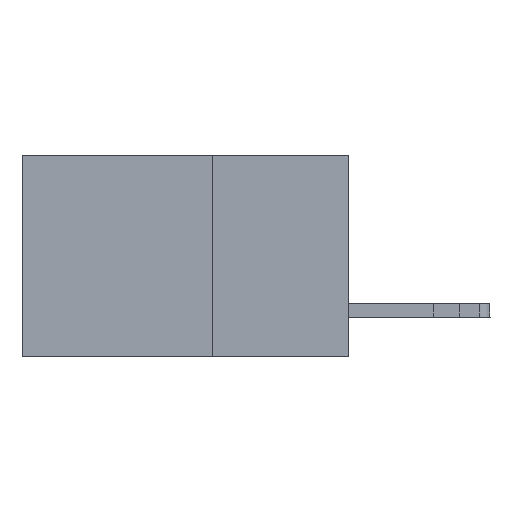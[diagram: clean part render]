
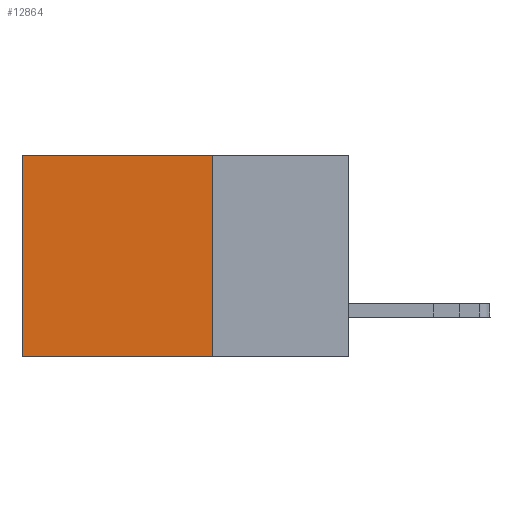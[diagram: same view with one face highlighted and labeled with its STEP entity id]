
A CAD part, left-side view. The second image highlights one B-rep face of the part: STEP entity #12864.
In plain terms, the highlighted planar face has unit normal (-1, 0, 0).
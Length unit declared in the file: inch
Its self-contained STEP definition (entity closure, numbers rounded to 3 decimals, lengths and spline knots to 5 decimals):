
#152 = CARTESIAN_POINT ( 'NONE',  ( 0.298, 0.25, 0. ) ) ;
#341 = DIRECTION ( 'NONE',  ( 0., 1., 0. ) ) ;
#676 = EDGE_CURVE ( 'NONE', #10019, #4765, #17692, .T. ) ;
#2193 = VECTOR ( 'NONE', #7711, 39.37008 ) ;
#2790 = EDGE_CURVE ( 'NONE', #4765, #21662, #24842, .T. ) ;
#4489 = EDGE_LOOP ( 'NONE', ( #12050, #15477, #16972, #23974 ) ) ;
#4526 = AXIS2_PLACEMENT_3D ( 'NONE', #23938, #21741, #7765 ) ;
#4765 = VERTEX_POINT ( 'NONE', #11971 ) ;
#5808 = EDGE_CURVE ( 'NONE', #10019, #13779, #13981, .T. ) ;
#6183 = CARTESIAN_POINT ( 'NONE',  ( 0.298, 0.6, -0.37 ) ) ;
#6931 = LINE ( 'NONE', #18487, #7171 ) ;
#7171 = VECTOR ( 'NONE', #16794, 39.37008 ) ;
#7711 = DIRECTION ( 'NONE',  ( 0., 0., -1. ) ) ;
#7765 = DIRECTION ( 'NONE',  ( 0., 0., -1. ) ) ;
#10019 = VERTEX_POINT ( 'NONE', #21011 ) ;
#11971 = CARTESIAN_POINT ( 'NONE',  ( 0.298, 0.25, -0.37 ) ) ;
#12050 = ORIENTED_EDGE ( 'NONE', *, *, #24105, .T. ) ;
#12864 = ADVANCED_FACE ( 'NONE', ( #16037 ), #25641, .F. ) ;
#13779 = VERTEX_POINT ( 'NONE', #22524 ) ;
#13981 = LINE ( 'NONE', #20196, #16504 ) ;
#15477 = ORIENTED_EDGE ( 'NONE', *, *, #2790, .F. ) ;
#16037 = FACE_OUTER_BOUND ( 'NONE', #4489, .T. ) ;
#16409 = VECTOR ( 'NONE', #17212, 39.37008 ) ;
#16504 = VECTOR ( 'NONE', #341, 39.37008 ) ;
#16794 = DIRECTION ( 'NONE',  ( 0., 0., -1. ) ) ;
#16972 = ORIENTED_EDGE ( 'NONE', *, *, #676, .F. ) ;
#17212 = DIRECTION ( 'NONE',  ( 0., 1., 0. ) ) ;
#17692 = LINE ( 'NONE', #152, #2193 ) ;
#18487 = CARTESIAN_POINT ( 'NONE',  ( 0.298, 0.6, 0. ) ) ;
#20196 = CARTESIAN_POINT ( 'NONE',  ( 0.298, 0.25, 0. ) ) ;
#20834 = CARTESIAN_POINT ( 'NONE',  ( 0.298, 0.25, -0.37 ) ) ;
#21011 = CARTESIAN_POINT ( 'NONE',  ( 0.298, 0.25, 0. ) ) ;
#21662 = VERTEX_POINT ( 'NONE', #6183 ) ;
#21741 = DIRECTION ( 'NONE',  ( 1., 0., 0. ) ) ;
#22524 = CARTESIAN_POINT ( 'NONE',  ( 0.298, 0.6, 0. ) ) ;
#23938 = CARTESIAN_POINT ( 'NONE',  ( 0.298, 0.25, 0. ) ) ;
#23974 = ORIENTED_EDGE ( 'NONE', *, *, #5808, .T. ) ;
#24105 = EDGE_CURVE ( 'NONE', #13779, #21662, #6931, .T. ) ;
#24842 = LINE ( 'NONE', #20834, #16409 ) ;
#25641 = PLANE ( 'NONE',  #4526 ) ;
